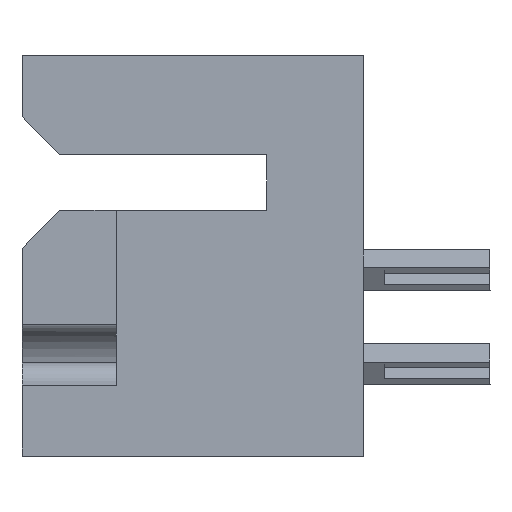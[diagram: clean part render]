
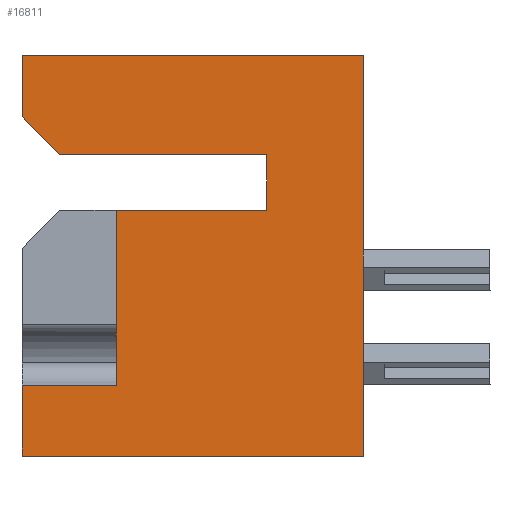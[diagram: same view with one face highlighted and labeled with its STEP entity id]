
A CAD part, left-side view. The second image highlights one B-rep face of the part: STEP entity #16811.
In plain terms, the highlighted planar face has unit normal (-1, 0, 0).
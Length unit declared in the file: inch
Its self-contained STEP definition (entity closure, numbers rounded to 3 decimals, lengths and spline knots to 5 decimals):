
#181 = CARTESIAN_POINT ( 'NONE',  ( 0., 0.403, -0.131 ) ) ;
#454 = VERTEX_POINT ( 'NONE', #17396 ) ;
#481 = VERTEX_POINT ( 'NONE', #19879 ) ;
#606 = VERTEX_POINT ( 'NONE', #20191 ) ;
#747 = ORIENTED_EDGE ( 'NONE', *, *, #11588, .F. ) ;
#753 = CARTESIAN_POINT ( 'NONE',  ( 0., 0.128, -0.131 ) ) ;
#835 = ORIENTED_EDGE ( 'NONE', *, *, #27903, .T. ) ;
#1088 = ORIENTED_EDGE ( 'NONE', *, *, #23487, .T. ) ;
#1111 = DIRECTION ( 'NONE',  ( 0., 0., 1. ) ) ;
#1123 = EDGE_CURVE ( 'NONE', #11621, #22717, #21165, .T. ) ;
#1126 = ORIENTED_EDGE ( 'NONE', *, *, #30448, .F. ) ;
#1409 = DIRECTION ( 'NONE',  ( 0., 0., 1. ) ) ;
#1825 = ORIENTED_EDGE ( 'NONE', *, *, #27891, .F. ) ;
#2044 = EDGE_CURVE ( 'NONE', #8376, #13477, #21108, .T. ) ;
#2586 = DIRECTION ( 'NONE',  ( 0., 1., 0. ) ) ;
#3017 = VERTEX_POINT ( 'NONE', #753 ) ;
#3214 = LINE ( 'NONE', #17756, #21022 ) ;
#3647 = DIRECTION ( 'NONE',  ( 0., -1., 0. ) ) ;
#3723 = DIRECTION ( 'NONE',  ( 0., -1., 0. ) ) ;
#3807 = ORIENTED_EDGE ( 'NONE', *, *, #1123, .F. ) ;
#3871 = VERTEX_POINT ( 'NONE', #181 ) ;
#4017 = EDGE_CURVE ( 'NONE', #481, #606, #7137, .T. ) ;
#4068 = EDGE_LOOP ( 'NONE', ( #835, #15404, #25189, #24158, #1825, #11352, #1088, #747, #1126, #26949, #3807 ) ) ;
#4842 = VERTEX_POINT ( 'NONE', #18707 ) ;
#5467 = EDGE_CURVE ( 'NONE', #481, #13883, #13414, .T. ) ;
#5471 = CARTESIAN_POINT ( 'NONE',  ( 0., 0.328, -0.205 ) ) ;
#6144 = AXIS2_PLACEMENT_3D ( 'NONE', #30436, #7000, #18632 ) ;
#6329 = CARTESIAN_POINT ( 'NONE',  ( 0., 0.453, 0. ) ) ;
#6512 = LINE ( 'NONE', #16818, #13580 ) ;
#7000 = DIRECTION ( 'NONE',  ( 1., 0., 0. ) ) ;
#7137 = LINE ( 'NONE', #12930, #12706 ) ;
#7773 = VECTOR ( 'NONE', #1111, 39.37008 ) ;
#8376 = VERTEX_POINT ( 'NONE', #27193 ) ;
#9220 = LINE ( 'NONE', #20072, #27109 ) ;
#9337 = VECTOR ( 'NONE', #20835, 39.37008 ) ;
#11352 = ORIENTED_EDGE ( 'NONE', *, *, #2044, .F. ) ;
#11588 = EDGE_CURVE ( 'NONE', #3017, #3871, #6512, .T. ) ;
#11621 = VERTEX_POINT ( 'NONE', #12848 ) ;
#12706 = VECTOR ( 'NONE', #1409, 39.37008 ) ;
#12848 = CARTESIAN_POINT ( 'NONE',  ( 0., 0.328, -0.437 ) ) ;
#12930 = CARTESIAN_POINT ( 'NONE',  ( 0., 0.453, 0. ) ) ;
#13414 = LINE ( 'NONE', #17939, #14150 ) ;
#13477 = VERTEX_POINT ( 'NONE', #6329 ) ;
#13580 = VECTOR ( 'NONE', #2586, 39.37008 ) ;
#13715 = FACE_OUTER_BOUND ( 'NONE', #4068, .T. ) ;
#13883 = VERTEX_POINT ( 'NONE', #17424 ) ;
#14112 = DIRECTION ( 'NONE',  ( 0., 1., 0. ) ) ;
#14150 = VECTOR ( 'NONE', #3723, 39.37008 ) ;
#14212 = CARTESIAN_POINT ( 'NONE',  ( 0., 0.128, -0.205 ) ) ;
#14348 = VECTOR ( 'NONE', #14112, 39.37008 ) ;
#14926 = CARTESIAN_POINT ( 'NONE',  ( 0., 0.453, 0. ) ) ;
#15404 = ORIENTED_EDGE ( 'NONE', *, *, #4017, .F. ) ;
#15490 = CARTESIAN_POINT ( 'NONE',  ( 0., 0.453, 0. ) ) ;
#16811 = ADVANCED_FACE ( 'NONE', ( #13715 ), #20831, .F. ) ;
#16818 = CARTESIAN_POINT ( 'NONE',  ( 0., 0.128, -0.131 ) ) ;
#17396 = CARTESIAN_POINT ( 'NONE',  ( 0., 0., 0. ) ) ;
#17424 = CARTESIAN_POINT ( 'NONE',  ( 0., 0., -0.531 ) ) ;
#17756 = CARTESIAN_POINT ( 'NONE',  ( 0., 0.328, -0.437 ) ) ;
#17772 = DIRECTION ( 'NONE',  ( 0., -0.707, -0.707 ) ) ;
#17813 = CARTESIAN_POINT ( 'NONE',  ( 0., 0.328, -0.205 ) ) ;
#17939 = CARTESIAN_POINT ( 'NONE',  ( 0., 0.453, -0.531 ) ) ;
#18124 = VECTOR ( 'NONE', #21675, 39.37008 ) ;
#18632 = DIRECTION ( 'NONE',  ( 0., 0., -1. ) ) ;
#18707 = CARTESIAN_POINT ( 'NONE',  ( 0., 0.128, -0.205 ) ) ;
#19134 = EDGE_CURVE ( 'NONE', #4842, #22717, #19172, .T. ) ;
#19172 = LINE ( 'NONE', #14212, #14348 ) ;
#19879 = CARTESIAN_POINT ( 'NONE',  ( 0., 0.453, -0.531 ) ) ;
#20072 = CARTESIAN_POINT ( 'NONE',  ( 0., 0.403, -0.131 ) ) ;
#20191 = CARTESIAN_POINT ( 'NONE',  ( 0., 0.453, -0.437 ) ) ;
#20483 = LINE ( 'NONE', #25516, #9337 ) ;
#20676 = LINE ( 'NONE', #15490, #22172 ) ;
#20831 = PLANE ( 'NONE',  #6144 ) ;
#20835 = DIRECTION ( 'NONE',  ( 0., 0., 1. ) ) ;
#21022 = VECTOR ( 'NONE', #25054, 39.37008 ) ;
#21108 = LINE ( 'NONE', #14926, #18124 ) ;
#21165 = LINE ( 'NONE', #17813, #7773 ) ;
#21566 = DIRECTION ( 'NONE',  ( 0., 0., 1. ) ) ;
#21675 = DIRECTION ( 'NONE',  ( 0., 0., 1. ) ) ;
#22172 = VECTOR ( 'NONE', #3647, 39.37008 ) ;
#22717 = VERTEX_POINT ( 'NONE', #5471 ) ;
#23487 = EDGE_CURVE ( 'NONE', #8376, #3871, #9220, .T. ) ;
#23580 = VECTOR ( 'NONE', #21566, 39.37008 ) ;
#24158 = ORIENTED_EDGE ( 'NONE', *, *, #28652, .T. ) ;
#25054 = DIRECTION ( 'NONE',  ( 0., 1., 0. ) ) ;
#25189 = ORIENTED_EDGE ( 'NONE', *, *, #5467, .T. ) ;
#25516 = CARTESIAN_POINT ( 'NONE',  ( 0., 0.128, -0.131 ) ) ;
#26278 = CARTESIAN_POINT ( 'NONE',  ( 0., 0., 0. ) ) ;
#26949 = ORIENTED_EDGE ( 'NONE', *, *, #19134, .T. ) ;
#27109 = VECTOR ( 'NONE', #17772, 39.37008 ) ;
#27193 = CARTESIAN_POINT ( 'NONE',  ( 0., 0.453, -0.081 ) ) ;
#27891 = EDGE_CURVE ( 'NONE', #13477, #454, #20676, .T. ) ;
#27903 = EDGE_CURVE ( 'NONE', #11621, #606, #3214, .T. ) ;
#28652 = EDGE_CURVE ( 'NONE', #13883, #454, #29197, .T. ) ;
#29197 = LINE ( 'NONE', #26278, #23580 ) ;
#30436 = CARTESIAN_POINT ( 'NONE',  ( 0., 0.453, 0. ) ) ;
#30448 = EDGE_CURVE ( 'NONE', #4842, #3017, #20483, .T. ) ;
